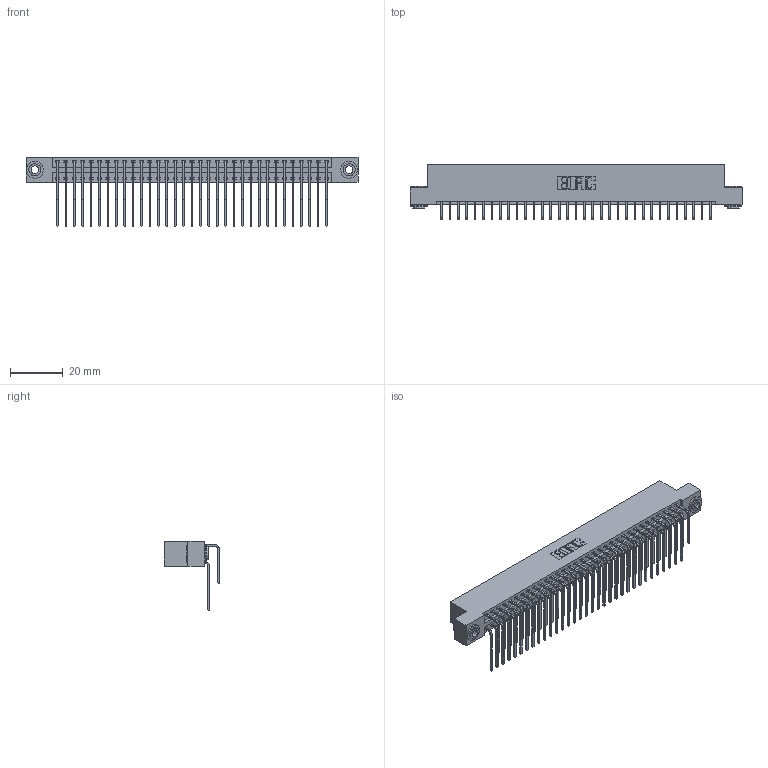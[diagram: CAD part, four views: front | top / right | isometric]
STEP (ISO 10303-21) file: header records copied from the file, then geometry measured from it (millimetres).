
FILE_DESCRIPTION (( 'STEP AP203' ), '1' );
FILE_NAME ('346-066-559-203.STEP', '2022-05-24T18:04:35', ( '' ), ( '' ), 'SwSTEP 2.0', 'SolidWorks 2020', '' );
FILE_SCHEMA (( 'CONFIG_CONTROL_DESIGN' ));
Length unit declared in the file: inch
Products named in the file (5): 346-066-559-203; 345-292-001_559 Tail - 2; 346 Part_Flush Mounting Lugs - 0.156 Dia-TH; 345-250-002_345-250-002-102; 345-292-001_558 559 Tail - 1
Assembly tree (69 placements, depth 2):
  346-066-559-203
    346 Part_Flush Mounting Lugs - 0.156 Dia-TH
    345-292-001_558 559 Tail - 1  x33
    345-292-001_559 Tail - 2  x33
    345-250-002_345-250-002-102  x2
Bounding box: 125.35 x 20.89 x 26.16 mm (x, y, z)
Volume: 12535.2 mm3; surface area: 19164.3 mm2
Topology: 69 solids, 69 shells, 3738 faces, 11067 edges, 7286 vertices
Faces by surface type: plane 2542, cylinder 1188, cone 8
Entity records: 25598 total; most frequent: CARTESIAN_POINT 4264, ORIENTED_EDGE 4138, DIRECTION 3811, EDGE_CURVE 2069, LINE 1741, VECTOR 1741, VERTEX_POINT 1374, AXIS2_PLACEMENT_3D 1035
